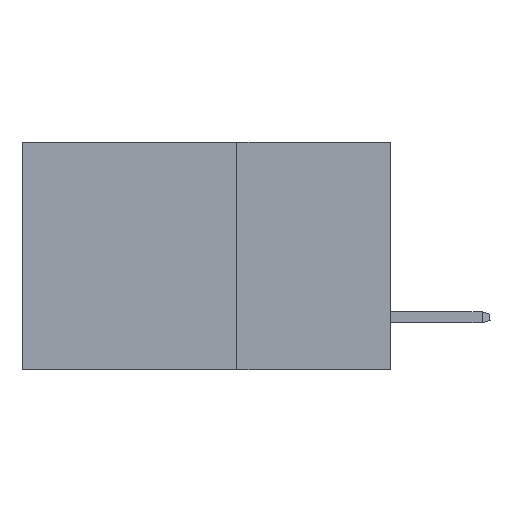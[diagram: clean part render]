
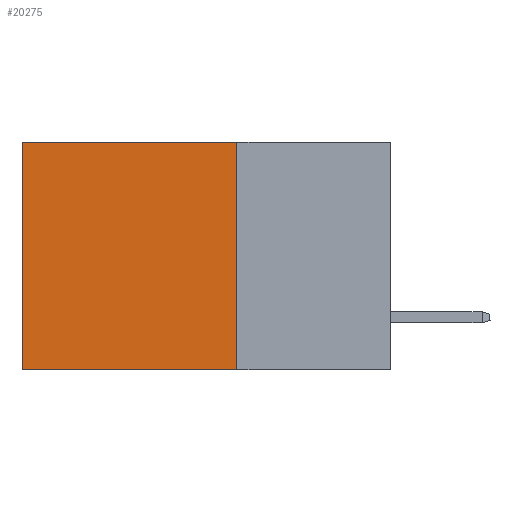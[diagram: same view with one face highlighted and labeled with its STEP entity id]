
A CAD part, left-side view. The second image highlights one B-rep face of the part: STEP entity #20275.
In plain terms, the highlighted planar face has unit normal (-1, 0, 0).
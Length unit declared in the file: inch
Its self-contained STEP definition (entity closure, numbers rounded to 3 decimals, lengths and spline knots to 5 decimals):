
#3144 = VECTOR ( 'NONE', #8407, 39.37008 ) ;
#3327 = FACE_OUTER_BOUND ( 'NONE', #23811, .T. ) ;
#3897 = LINE ( 'NONE', #9878, #10004 ) ;
#7288 = CARTESIAN_POINT ( 'NONE',  ( 0.2875, 0.6, 0. ) ) ;
#8407 = DIRECTION ( 'NONE',  ( 0., 0., -1. ) ) ;
#8616 = CARTESIAN_POINT ( 'NONE',  ( 0.2875, 0.25, 0. ) ) ;
#9551 = VECTOR ( 'NONE', #20818, 39.37008 ) ;
#9878 = CARTESIAN_POINT ( 'NONE',  ( 0.2875, 0.25, -0.37 ) ) ;
#10004 = VECTOR ( 'NONE', #23409, 39.37008 ) ;
#10667 = EDGE_CURVE ( 'NONE', #25901, #39908, #25261, .T. ) ;
#12641 = CARTESIAN_POINT ( 'NONE',  ( 0.2875, 0.25, 0. ) ) ;
#13945 = LINE ( 'NONE', #7288, #9551 ) ;
#14489 = DIRECTION ( 'NONE',  ( 0., 0., -1. ) ) ;
#15176 = ORIENTED_EDGE ( 'NONE', *, *, #31316, .F. ) ;
#16835 = DIRECTION ( 'NONE',  ( 1., 0., 0. ) ) ;
#19037 = EDGE_CURVE ( 'NONE', #38750, #43812, #13945, .T. ) ;
#19521 = LINE ( 'NONE', #12641, #27376 ) ;
#20275 = ADVANCED_FACE ( 'NONE', ( #3327 ), #24383, .F. ) ;
#20348 = ORIENTED_EDGE ( 'NONE', *, *, #21335, .T. ) ;
#20818 = DIRECTION ( 'NONE',  ( 0., 0., -1. ) ) ;
#21335 = EDGE_CURVE ( 'NONE', #25901, #38750, #19521, .T. ) ;
#23282 = DIRECTION ( 'NONE',  ( 0., 1., 0. ) ) ;
#23409 = DIRECTION ( 'NONE',  ( 0., 1., 0. ) ) ;
#23811 = EDGE_LOOP ( 'NONE', ( #36522, #15176, #25131, #20348 ) ) ;
#24383 = PLANE ( 'NONE',  #37935 ) ;
#25131 = ORIENTED_EDGE ( 'NONE', *, *, #10667, .F. ) ;
#25261 = LINE ( 'NONE', #8616, #3144 ) ;
#25901 = VERTEX_POINT ( 'NONE', #43393 ) ;
#27376 = VECTOR ( 'NONE', #23282, 39.37008 ) ;
#30084 = CARTESIAN_POINT ( 'NONE',  ( 0.2875, 0.25, -0.37 ) ) ;
#30729 = CARTESIAN_POINT ( 'NONE',  ( 0.2875, 0.6, 0. ) ) ;
#31316 = EDGE_CURVE ( 'NONE', #39908, #43812, #3897, .T. ) ;
#36522 = ORIENTED_EDGE ( 'NONE', *, *, #19037, .T. ) ;
#37935 = AXIS2_PLACEMENT_3D ( 'NONE', #41019, #16835, #14489 ) ;
#38750 = VERTEX_POINT ( 'NONE', #30729 ) ;
#39908 = VERTEX_POINT ( 'NONE', #30084 ) ;
#41019 = CARTESIAN_POINT ( 'NONE',  ( 0.2875, 0.25, 0. ) ) ;
#42960 = CARTESIAN_POINT ( 'NONE',  ( 0.2875, 0.6, -0.37 ) ) ;
#43393 = CARTESIAN_POINT ( 'NONE',  ( 0.2875, 0.25, 0. ) ) ;
#43812 = VERTEX_POINT ( 'NONE', #42960 ) ;
